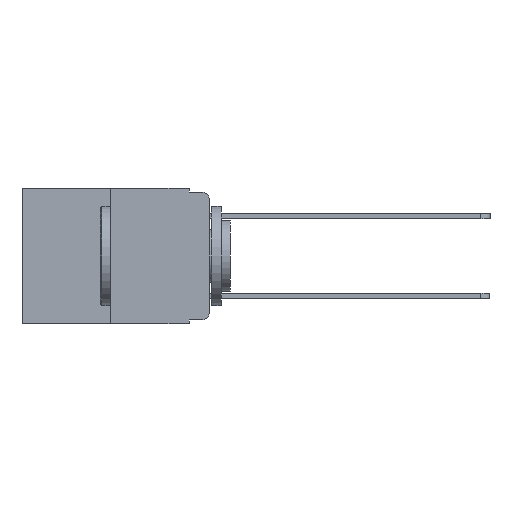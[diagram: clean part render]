
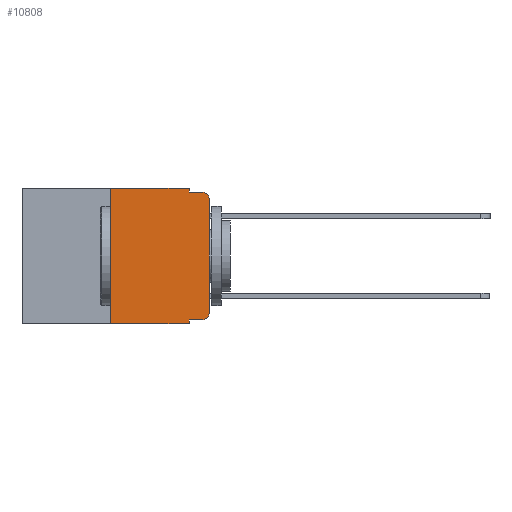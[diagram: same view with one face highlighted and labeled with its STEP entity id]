
A CAD part, left-side view. The second image highlights one B-rep face of the part: STEP entity #10808.
In plain terms, the highlighted planar face has unit normal (-1, 0, 0).
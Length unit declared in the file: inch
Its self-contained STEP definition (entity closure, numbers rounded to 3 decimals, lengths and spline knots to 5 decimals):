
#44 = VERTEX_POINT ( 'NONE', #10527 ) ;
#311 = PLANE ( 'NONE',  #3863 ) ;
#648 = CARTESIAN_POINT ( 'NONE',  ( 0., 0., -0.03 ) ) ;
#1355 = EDGE_LOOP ( 'NONE', ( #14392, #18120, #14572, #15806, #9721, #14314, #13855, #17756, #9439, #7497 ) ) ;
#1894 = VERTEX_POINT ( 'NONE', #17680 ) ;
#2070 = EDGE_CURVE ( 'NONE', #18574, #14728, #20683, .T. ) ;
#2102 = EDGE_CURVE ( 'NONE', #14728, #19916, #16226, .T. ) ;
#2124 = EDGE_CURVE ( 'NONE', #18574, #4083, #19282, .T. ) ;
#2198 = DIRECTION ( 'NONE',  ( 1., 0., 0. ) ) ;
#2462 = CARTESIAN_POINT ( 'NONE',  ( 0., 0.473, -0.343 ) ) ;
#3213 = DIRECTION ( 'NONE',  ( 0., 0., 1. ) ) ;
#3408 = VECTOR ( 'NONE', #12859, 39.37008 ) ;
#3538 = DIRECTION ( 'NONE',  ( 0., 0., -1. ) ) ;
#3863 = AXIS2_PLACEMENT_3D ( 'NONE', #10359, #2198, #13520 ) ;
#4083 = VERTEX_POINT ( 'NONE', #20643 ) ;
#4121 = EDGE_CURVE ( 'NONE', #15228, #7880, #20598, .T. ) ;
#4311 = CARTESIAN_POINT ( 'NONE',  ( 0., 0.02, -0.03 ) ) ;
#4700 = LINE ( 'NONE', #12836, #19815 ) ;
#4897 = CARTESIAN_POINT ( 'NONE',  ( 0., 0.051, 0. ) ) ;
#5280 = LINE ( 'NONE', #18210, #9526 ) ;
#5341 = CARTESIAN_POINT ( 'NONE',  ( 0., 0.051, -0.333 ) ) ;
#5383 = EDGE_CURVE ( 'NONE', #15228, #4083, #12265, .T. ) ;
#5436 = CARTESIAN_POINT ( 'NONE',  ( 0., 0.02, -0.01 ) ) ;
#6014 = DIRECTION ( 'NONE',  ( 0., 0., -1. ) ) ;
#6929 = VECTOR ( 'NONE', #12272, 39.37008 ) ;
#7118 = CARTESIAN_POINT ( 'NONE',  ( 0., 0.051, -0.01 ) ) ;
#7497 = ORIENTED_EDGE ( 'NONE', *, *, #2102, .T. ) ;
#7747 = LINE ( 'NONE', #15821, #3408 ) ;
#7880 = VERTEX_POINT ( 'NONE', #14771 ) ;
#8317 = VECTOR ( 'NONE', #14710, 39.37008 ) ;
#8413 = VECTOR ( 'NONE', #10387, 39.37008 ) ;
#9439 = ORIENTED_EDGE ( 'NONE', *, *, #2070, .T. ) ;
#9526 = VECTOR ( 'NONE', #15169, 39.37008 ) ;
#9721 = ORIENTED_EDGE ( 'NONE', *, *, #18814, .F. ) ;
#10203 = EDGE_CURVE ( 'NONE', #18072, #19463, #17308, .T. ) ;
#10359 = CARTESIAN_POINT ( 'NONE',  ( 0., 0.473, 0. ) ) ;
#10387 = DIRECTION ( 'NONE',  ( 0., -1., 0. ) ) ;
#10527 = CARTESIAN_POINT ( 'NONE',  ( 0., 0.051, -0.01 ) ) ;
#10808 = ADVANCED_FACE ( 'NONE', ( #19850 ), #311, .F. ) ;
#12173 = DIRECTION ( 'NONE',  ( 0., -1., 0. ) ) ;
#12265 = LINE ( 'NONE', #2462, #16341 ) ;
#12272 = DIRECTION ( 'NONE',  ( 0., 0., -1. ) ) ;
#12432 = LINE ( 'NONE', #7118, #16515 ) ;
#12492 = EDGE_CURVE ( 'NONE', #19916, #18072, #4700, .T. ) ;
#12836 = CARTESIAN_POINT ( 'NONE',  ( 0., 0., 0. ) ) ;
#12859 = DIRECTION ( 'NONE',  ( 0., 0., -1. ) ) ;
#13164 = CARTESIAN_POINT ( 'NONE',  ( 0., 0.25, 0. ) ) ;
#13423 = CARTESIAN_POINT ( 'NONE',  ( 0., 0., -0.313 ) ) ;
#13520 = DIRECTION ( 'NONE',  ( 0., 0., -1. ) ) ;
#13855 = ORIENTED_EDGE ( 'NONE', *, *, #5383, .T. ) ;
#14314 = ORIENTED_EDGE ( 'NONE', *, *, #4121, .F. ) ;
#14392 = ORIENTED_EDGE ( 'NONE', *, *, #12492, .T. ) ;
#14572 = ORIENTED_EDGE ( 'NONE', *, *, #15160, .F. ) ;
#14710 = DIRECTION ( 'NONE',  ( 0., 0., 1. ) ) ;
#14728 = VERTEX_POINT ( 'NONE', #19689 ) ;
#14771 = CARTESIAN_POINT ( 'NONE',  ( 0., 0.25, 0. ) ) ;
#15153 = CARTESIAN_POINT ( 'NONE',  ( 0., 0.02, -0.313 ) ) ;
#15160 = EDGE_CURVE ( 'NONE', #44, #19463, #12432, .T. ) ;
#15169 = DIRECTION ( 'NONE',  ( 0., -1., 0. ) ) ;
#15228 = VERTEX_POINT ( 'NONE', #18141 ) ;
#15295 = AXIS2_PLACEMENT_3D ( 'NONE', #4311, #15407, #6014 ) ;
#15407 = DIRECTION ( 'NONE',  ( -1., 0., 0. ) ) ;
#15806 = ORIENTED_EDGE ( 'NONE', *, *, #19201, .F. ) ;
#15821 = CARTESIAN_POINT ( 'NONE',  ( 0., 0.051, 0. ) ) ;
#16226 = CIRCLE ( 'NONE', #17366, 0.02 ) ;
#16341 = VECTOR ( 'NONE', #12173, 39.37008 ) ;
#16515 = VECTOR ( 'NONE', #18019, 39.37008 ) ;
#17308 = CIRCLE ( 'NONE', #15295, 0.02 ) ;
#17366 = AXIS2_PLACEMENT_3D ( 'NONE', #15153, #18194, #3538 ) ;
#17680 = CARTESIAN_POINT ( 'NONE',  ( 0., 0.051, 0. ) ) ;
#17703 = CARTESIAN_POINT ( 'NONE',  ( 0., 0.051, -0.333 ) ) ;
#17756 = ORIENTED_EDGE ( 'NONE', *, *, #2124, .F. ) ;
#18019 = DIRECTION ( 'NONE',  ( 0., -1., 0. ) ) ;
#18072 = VERTEX_POINT ( 'NONE', #648 ) ;
#18120 = ORIENTED_EDGE ( 'NONE', *, *, #10203, .T. ) ;
#18141 = CARTESIAN_POINT ( 'NONE',  ( 0., 0.25, -0.343 ) ) ;
#18194 = DIRECTION ( 'NONE',  ( -1., 0., 0. ) ) ;
#18210 = CARTESIAN_POINT ( 'NONE',  ( 0., 0.473, 0. ) ) ;
#18574 = VERTEX_POINT ( 'NONE', #17703 ) ;
#18814 = EDGE_CURVE ( 'NONE', #7880, #1894, #5280, .T. ) ;
#19201 = EDGE_CURVE ( 'NONE', #1894, #44, #7747, .T. ) ;
#19282 = LINE ( 'NONE', #4897, #6929 ) ;
#19463 = VERTEX_POINT ( 'NONE', #5436 ) ;
#19689 = CARTESIAN_POINT ( 'NONE',  ( 0., 0.02, -0.333 ) ) ;
#19815 = VECTOR ( 'NONE', #3213, 39.37008 ) ;
#19850 = FACE_OUTER_BOUND ( 'NONE', #1355, .T. ) ;
#19916 = VERTEX_POINT ( 'NONE', #13423 ) ;
#20598 = LINE ( 'NONE', #13164, #8317 ) ;
#20643 = CARTESIAN_POINT ( 'NONE',  ( 0., 0.051, -0.343 ) ) ;
#20683 = LINE ( 'NONE', #5341, #8413 ) ;
